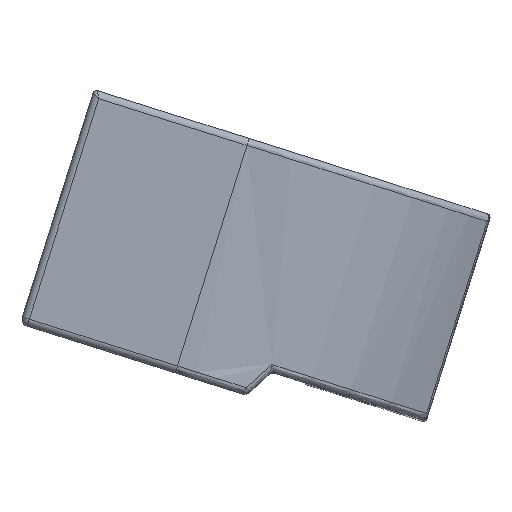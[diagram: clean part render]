
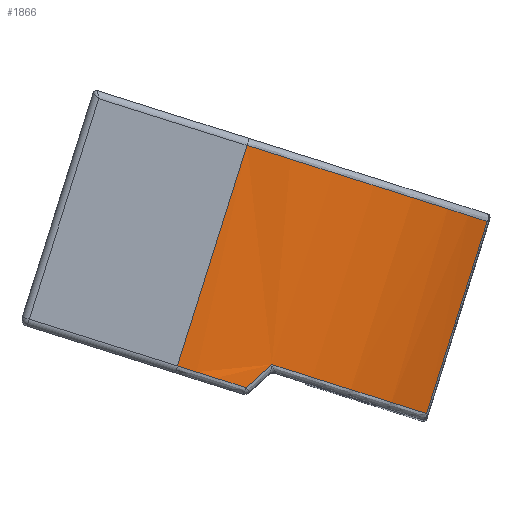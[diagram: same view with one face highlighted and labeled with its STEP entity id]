
A CAD part, top view. The second image highlights one B-rep face of the part: STEP entity #1866.
In plain terms, the highlighted free-form (B-spline) face has degree [3, 1] with [15, 2] control points.
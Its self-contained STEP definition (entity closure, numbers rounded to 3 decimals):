
#26=(
BOUNDED_SURFACE()
B_SPLINE_SURFACE(3,1,((#3465,#3466),(#3467,#3468),(#3469,#3470),(#3471,
#3472),(#3473,#3474),(#3475,#3476),(#3477,#3478),(#3479,#3480),(#3481,#3482),
(#3483,#3484),(#3485,#3486),(#3487,#3488),(#3489,#3490),(#3491,#3492),(#3493,
#3494)),.UNSPECIFIED.,.F.,.F.,.F.)
B_SPLINE_SURFACE_WITH_KNOTS((4,2,2,2,3,2,4),(2,2),(-1.571,-1.456,
-1.342,-1.228,-1.113,-0.885,
-0.656),(0.,0.848),.UNSPECIFIED.)
GEOMETRIC_REPRESENTATION_ITEM()
RATIONAL_B_SPLINE_SURFACE(((1.,1.),(1.,1.),(1.,1.),(1.,1.),(1.,1.),(1.,
1.),(1.,1.),(1.,1.),(1.,1.),(1.,1.),(1.,1.),(1.,1.),(1.,1.),(1.,1.),(1.,
1.)))
REPRESENTATION_ITEM('')
SURFACE()
);
#126=LINE('',#3464,#260);
#260=VECTOR('',#2343,10.);
#429=FACE_OUTER_BOUND('',#552,.T.);
#552=EDGE_LOOP('',(#1403,#1404,#1405,#1406,#1407,#1408));
#651=B_SPLINE_CURVE_WITH_KNOTS('',3,(#2893,#2894,#2895,#2896,#2897,#2898),
 .UNSPECIFIED.,.F.,.F.,(4,2,4),(-0.148,-0.039,-0.029),
 .UNSPECIFIED.);
#653=B_SPLINE_CURVE_WITH_KNOTS('',3,(#2976,#2977,#2978,#2979,#2980,#2981),
 .UNSPECIFIED.,.F.,.F.,(4,2,4),(-0.243,-0.124,0.),
 .UNSPECIFIED.);
#663=B_SPLINE_CURVE_WITH_KNOTS('',3,(#3224,#3225,#3226,#3227,#3228,#3229,
#3230,#3231,#3232,#3233),.UNSPECIFIED.,.F.,.F.,(4,2,2,2,4),(-0.968,
-0.747,-0.498,-0.374,-0.305),
 .UNSPECIFIED.);
#665=B_SPLINE_CURVE_WITH_KNOTS('',3,(#3328,#3329,#3330,#3331,#3332,#3333,
#3334,#3335,#3336,#3337,#3338,#3339,#3340,#3341),.UNSPECIFIED.,.F.,.F.,
(4,2,2,2,2,2,4),(-0.975,-0.851,-0.727,
-0.603,-0.478,-0.23,-0.009),
 .UNSPECIFIED.);
#667=B_SPLINE_CURVE_WITH_KNOTS('',3,(#3362,#3363,#3364,#3365),
 .UNSPECIFIED.,.F.,.F.,(4,4),(0.025,0.72),
 .UNSPECIFIED.);
#795=VERTEX_POINT('',#2801);
#802=VERTEX_POINT('',#2892);
#816=VERTEX_POINT('',#2975);
#821=VERTEX_POINT('',#3048);
#826=VERTEX_POINT('',#3126);
#829=VERTEX_POINT('',#3239);
#972=EDGE_CURVE('',#795,#802,#651,.T.);
#994=EDGE_CURVE('',#802,#816,#653,.T.);
#1012=EDGE_CURVE('',#821,#795,#663,.T.);
#1019=EDGE_CURVE('',#829,#826,#665,.T.);
#1021=EDGE_CURVE('',#826,#821,#667,.T.);
#1060=EDGE_CURVE('',#829,#816,#126,.T.);
#1403=ORIENTED_EDGE('',*,*,#1019,.F.);
#1404=ORIENTED_EDGE('',*,*,#1060,.T.);
#1405=ORIENTED_EDGE('',*,*,#994,.F.);
#1406=ORIENTED_EDGE('',*,*,#972,.F.);
#1407=ORIENTED_EDGE('',*,*,#1012,.F.);
#1408=ORIENTED_EDGE('',*,*,#1021,.F.);
#1866=ADVANCED_FACE('',(#429),#26,.F.);
#2343=DIRECTION('',(-0.301,-0.954,0.));
#2801=CARTESIAN_POINT('',(55.199,-39.499,13.82));
#2892=CARTESIAN_POINT('',(54.313,-40.295,13.976));
#2893=CARTESIAN_POINT('Ctrl Pts',(55.199,-39.499,13.82));
#2894=CARTESIAN_POINT('Ctrl Pts',(54.929,-39.741,13.873));
#2895=CARTESIAN_POINT('Ctrl Pts',(54.659,-39.984,13.921));
#2896=CARTESIAN_POINT('Ctrl Pts',(54.364,-40.249,13.968));
#2897=CARTESIAN_POINT('Ctrl Pts',(54.338,-40.272,13.972));
#2898=CARTESIAN_POINT('Ctrl Pts',(54.313,-40.295,13.976));
#2975=CARTESIAN_POINT('',(51.944,-39.548,14.255));
#2976=CARTESIAN_POINT('Ctrl Pts',(54.313,-40.295,13.976));
#2977=CARTESIAN_POINT('Ctrl Pts',(53.933,-40.175,14.066));
#2978=CARTESIAN_POINT('Ctrl Pts',(53.548,-40.053,14.135));
#2979=CARTESIAN_POINT('Ctrl Pts',(52.756,-39.803,14.231));
#2980=CARTESIAN_POINT('Ctrl Pts',(52.349,-39.675,14.255));
#2981=CARTESIAN_POINT('Ctrl Pts',(51.944,-39.548,14.255));
#3048=CARTESIAN_POINT('',(60.535,-41.182,10.121));
#3126=CARTESIAN_POINT('',(62.625,-34.553,10.121));
#3224=CARTESIAN_POINT('Ctrl Pts',(60.535,-41.182,10.121));
#3225=CARTESIAN_POINT('Ctrl Pts',(60.082,-41.039,10.705));
#3226=CARTESIAN_POINT('Ctrl Pts',(59.57,-40.877,11.245));
#3227=CARTESIAN_POINT('Ctrl Pts',(58.381,-40.502,12.265));
#3228=CARTESIAN_POINT('Ctrl Pts',(57.697,-40.287,12.727));
#3229=CARTESIAN_POINT('Ctrl Pts',(56.599,-39.941,13.293));
#3230=CARTESIAN_POINT('Ctrl Pts',(56.224,-39.822,13.46));
#3231=CARTESIAN_POINT('Ctrl Pts',(55.629,-39.635,13.683));
#3232=CARTESIAN_POINT('Ctrl Pts',(55.415,-39.567,13.755));
#3233=CARTESIAN_POINT('Ctrl Pts',(55.199,-39.499,13.82));
#3239=CARTESIAN_POINT('',(54.342,-31.942,14.255));
#3328=CARTESIAN_POINT('Ctrl Pts',(54.342,-31.942,14.255));
#3329=CARTESIAN_POINT('Ctrl Pts',(54.747,-32.069,14.255));
#3330=CARTESIAN_POINT('Ctrl Pts',(55.154,-32.198,14.231));
#3331=CARTESIAN_POINT('Ctrl Pts',(55.963,-32.453,14.133));
#3332=CARTESIAN_POINT('Ctrl Pts',(56.364,-32.579,14.06));
#3333=CARTESIAN_POINT('Ctrl Pts',(57.158,-32.829,13.867));
#3334=CARTESIAN_POINT('Ctrl Pts',(57.549,-32.953,13.746));
#3335=CARTESIAN_POINT('Ctrl Pts',(58.314,-33.194,13.46));
#3336=CARTESIAN_POINT('Ctrl Pts',(58.688,-33.312,13.294));
#3337=CARTESIAN_POINT('Ctrl Pts',(59.782,-33.657,12.73));
#3338=CARTESIAN_POINT('Ctrl Pts',(60.473,-33.875,12.263));
#3339=CARTESIAN_POINT('Ctrl Pts',(61.662,-34.25,11.243));
#3340=CARTESIAN_POINT('Ctrl Pts',(62.171,-34.41,10.706));
#3341=CARTESIAN_POINT('Ctrl Pts',(62.625,-34.553,10.121));
#3362=CARTESIAN_POINT('Ctrl Pts',(62.625,-34.553,10.121));
#3363=CARTESIAN_POINT('Ctrl Pts',(61.928,-36.763,10.121));
#3364=CARTESIAN_POINT('Ctrl Pts',(61.232,-38.972,10.121));
#3365=CARTESIAN_POINT('Ctrl Pts',(60.535,-41.182,10.121));
#3464=CARTESIAN_POINT('',(54.417,-31.703,14.255));
#3465=CARTESIAN_POINT('Ctrl Pts',(54.417,-31.703,14.255));
#3466=CARTESIAN_POINT('Ctrl Pts',(51.869,-39.786,14.255));
#3467=CARTESIAN_POINT('Ctrl Pts',(54.824,-31.831,14.255));
#3468=CARTESIAN_POINT('Ctrl Pts',(52.275,-39.914,14.255));
#3469=CARTESIAN_POINT('Ctrl Pts',(55.23,-31.96,14.23));
#3470=CARTESIAN_POINT('Ctrl Pts',(52.682,-40.042,14.23));
#3471=CARTESIAN_POINT('Ctrl Pts',(56.038,-32.214,14.133));
#3472=CARTESIAN_POINT('Ctrl Pts',(53.49,-40.297,14.133));
#3473=CARTESIAN_POINT('Ctrl Pts',(56.44,-32.341,14.06));
#3474=CARTESIAN_POINT('Ctrl Pts',(53.891,-40.424,14.06));
#3475=CARTESIAN_POINT('Ctrl Pts',(57.232,-32.591,13.867));
#3476=CARTESIAN_POINT('Ctrl Pts',(54.683,-40.673,13.867));
#3477=CARTESIAN_POINT('Ctrl Pts',(57.623,-32.714,13.747));
#3478=CARTESIAN_POINT('Ctrl Pts',(55.074,-40.797,13.747));
#3479=CARTESIAN_POINT('Ctrl Pts',(58.389,-32.955,13.46));
#3480=CARTESIAN_POINT('Ctrl Pts',(55.84,-41.038,13.46));
#3481=CARTESIAN_POINT('Ctrl Pts',(58.764,-33.074,13.293));
#3482=CARTESIAN_POINT('Ctrl Pts',(56.216,-41.157,13.293));
#3483=CARTESIAN_POINT('Ctrl Pts',(59.129,-33.189,13.105));
#3484=CARTESIAN_POINT('Ctrl Pts',(56.58,-41.272,13.105));
#3485=CARTESIAN_POINT('Ctrl Pts',(59.859,-33.419,12.729));
#3486=CARTESIAN_POINT('Ctrl Pts',(57.31,-41.502,12.729));
#3487=CARTESIAN_POINT('Ctrl Pts',(60.547,-33.636,12.264));
#3488=CARTESIAN_POINT('Ctrl Pts',(57.999,-41.719,12.264));
#3489=CARTESIAN_POINT('Ctrl Pts',(61.806,-34.033,11.184));
#3490=CARTESIAN_POINT('Ctrl Pts',(59.258,-42.116,11.184));
#3491=CARTESIAN_POINT('Ctrl Pts',(62.377,-34.213,10.568));
#3492=CARTESIAN_POINT('Ctrl Pts',(59.828,-42.296,10.568));
#3493=CARTESIAN_POINT('Ctrl Pts',(62.873,-34.369,9.892));
#3494=CARTESIAN_POINT('Ctrl Pts',(60.324,-42.452,9.892));
